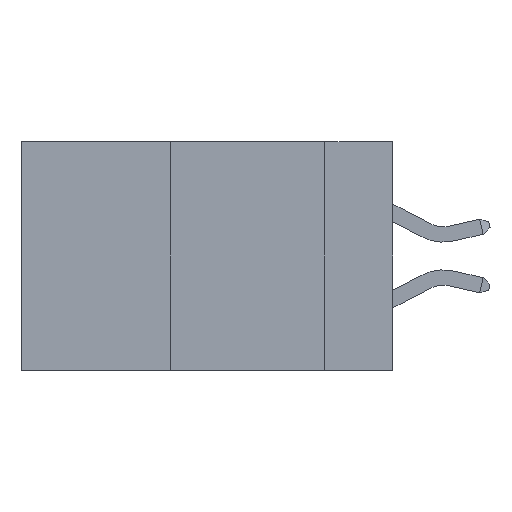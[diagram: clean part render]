
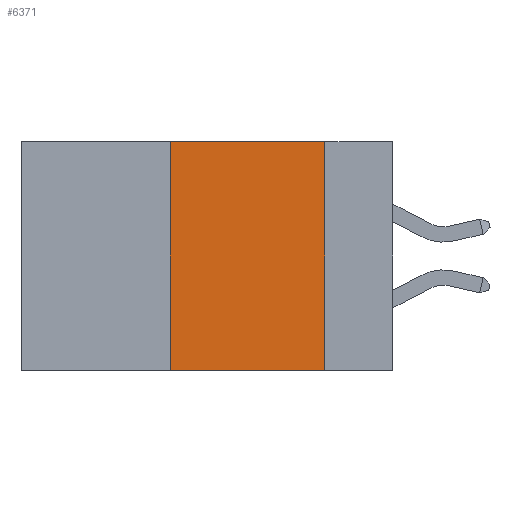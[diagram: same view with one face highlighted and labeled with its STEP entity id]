
A CAD part, left-side view. The second image highlights one B-rep face of the part: STEP entity #6371.
In plain terms, the highlighted planar face has unit normal (-1, 0, 0).
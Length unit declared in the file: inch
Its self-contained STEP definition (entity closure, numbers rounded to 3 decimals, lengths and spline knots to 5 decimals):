
#128 = DIRECTION ( 'NONE',  ( 0., 0., 1. ) ) ;
#262 = ORIENTED_EDGE ( 'NONE', *, *, #5851, .F. ) ;
#1217 = VERTEX_POINT ( 'NONE', #6082 ) ;
#1277 = DIRECTION ( 'NONE',  ( 1., 0., 0. ) ) ;
#1288 = ORIENTED_EDGE ( 'NONE', *, *, #12199, .T. ) ;
#1478 = CARTESIAN_POINT ( 'NONE',  ( 0., 0.36, 0. ) ) ;
#1507 = VERTEX_POINT ( 'NONE', #6731 ) ;
#1671 = LINE ( 'NONE', #1478, #2523 ) ;
#2523 = VECTOR ( 'NONE', #128, 39.37008 ) ;
#3011 = VECTOR ( 'NONE', #3209, 39.37008 ) ;
#3209 = DIRECTION ( 'NONE',  ( 0., -1., 0. ) ) ;
#4207 = CARTESIAN_POINT ( 'NONE',  ( 0., 0.6, 0. ) ) ;
#5470 = VERTEX_POINT ( 'NONE', #13539 ) ;
#5617 = CARTESIAN_POINT ( 'NONE',  ( 0., 0.6, -0.37 ) ) ;
#5851 = EDGE_CURVE ( 'NONE', #1507, #5470, #1671, .T. ) ;
#6082 = CARTESIAN_POINT ( 'NONE',  ( 0., 0.11, -0.37 ) ) ;
#6136 = ORIENTED_EDGE ( 'NONE', *, *, #16212, .F. ) ;
#6371 = ADVANCED_FACE ( 'NONE', ( #16883 ), #12635, .F. ) ;
#6410 = VERTEX_POINT ( 'NONE', #11138 ) ;
#6731 = CARTESIAN_POINT ( 'NONE',  ( 0., 0.36, -0.37 ) ) ;
#6734 = DIRECTION ( 'NONE',  ( 0., 0., -1. ) ) ;
#6814 = ORIENTED_EDGE ( 'NONE', *, *, #11208, .F. ) ;
#7033 = DIRECTION ( 'NONE',  ( 0., -1., 0. ) ) ;
#7214 = EDGE_LOOP ( 'NONE', ( #6136, #6814, #262, #1288 ) ) ;
#9985 = CARTESIAN_POINT ( 'NONE',  ( 0., 0.11, 0. ) ) ;
#11138 = CARTESIAN_POINT ( 'NONE',  ( 0., 0.11, 0. ) ) ;
#11208 = EDGE_CURVE ( 'NONE', #5470, #6410, #12239, .T. ) ;
#12199 = EDGE_CURVE ( 'NONE', #1507, #1217, #14677, .T. ) ;
#12239 = LINE ( 'NONE', #13175, #3011 ) ;
#12315 = LINE ( 'NONE', #9985, #15904 ) ;
#12318 = AXIS2_PLACEMENT_3D ( 'NONE', #4207, #1277, #6734 ) ;
#12635 = PLANE ( 'NONE',  #12318 ) ;
#13175 = CARTESIAN_POINT ( 'NONE',  ( 0., 0.6, 0. ) ) ;
#13539 = CARTESIAN_POINT ( 'NONE',  ( 0., 0.36, 0. ) ) ;
#13565 = VECTOR ( 'NONE', #7033, 39.37008 ) ;
#14677 = LINE ( 'NONE', #5617, #13565 ) ;
#15904 = VECTOR ( 'NONE', #17251, 39.37008 ) ;
#16212 = EDGE_CURVE ( 'NONE', #6410, #1217, #12315, .T. ) ;
#16883 = FACE_OUTER_BOUND ( 'NONE', #7214, .T. ) ;
#17251 = DIRECTION ( 'NONE',  ( 0., 0., -1. ) ) ;
